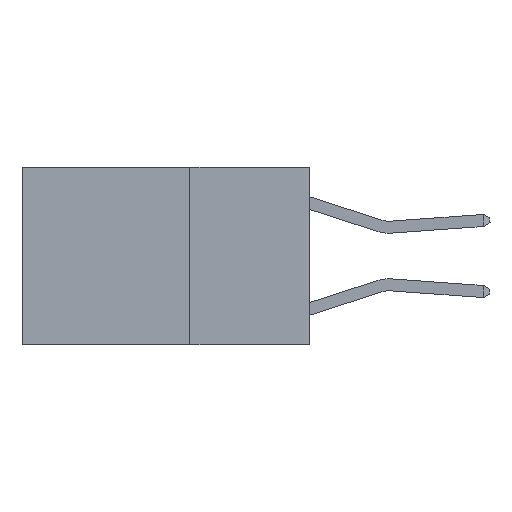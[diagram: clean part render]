
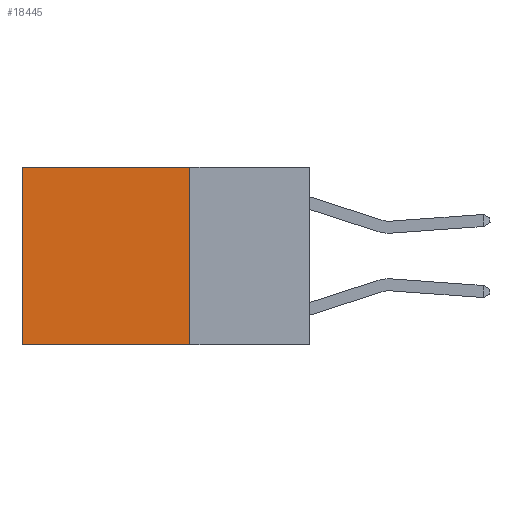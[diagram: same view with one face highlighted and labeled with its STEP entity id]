
A CAD part, left-side view. The second image highlights one B-rep face of the part: STEP entity #18445.
In plain terms, the highlighted planar face has unit normal (-1, 0, 0).
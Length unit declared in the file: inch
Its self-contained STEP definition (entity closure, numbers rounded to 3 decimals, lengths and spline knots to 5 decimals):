
#543 = LINE ( 'NONE', #3428, #13160 ) ;
#1810 = VECTOR ( 'NONE', #3182, 39.37008 ) ;
#2720 = ORIENTED_EDGE ( 'NONE', *, *, #27945, .F. ) ;
#2787 = CARTESIAN_POINT ( 'NONE',  ( 0.2625, 0.6, 0. ) ) ;
#3105 = CARTESIAN_POINT ( 'NONE',  ( 0.2625, 0.6, -0.37 ) ) ;
#3182 = DIRECTION ( 'NONE',  ( 0., 0., -1. ) ) ;
#3428 = CARTESIAN_POINT ( 'NONE',  ( 0.2625, 0.25, 0. ) ) ;
#3459 = PLANE ( 'NONE',  #4349 ) ;
#4349 = AXIS2_PLACEMENT_3D ( 'NONE', #16695, #25955, #12263 ) ;
#5688 = DIRECTION ( 'NONE',  ( 0., 1., 0. ) ) ;
#6063 = EDGE_LOOP ( 'NONE', ( #16466, #2720, #22241, #25282 ) ) ;
#7013 = LINE ( 'NONE', #18595, #1810 ) ;
#7098 = VERTEX_POINT ( 'NONE', #15454 ) ;
#8985 = CARTESIAN_POINT ( 'NONE',  ( 0.2625, 0.25, -0.37 ) ) ;
#10956 = VECTOR ( 'NONE', #25641, 39.37008 ) ;
#12170 = VERTEX_POINT ( 'NONE', #20185 ) ;
#12263 = DIRECTION ( 'NONE',  ( 0., 0., -1. ) ) ;
#12449 = EDGE_CURVE ( 'NONE', #7098, #12170, #22782, .T. ) ;
#13127 = VERTEX_POINT ( 'NONE', #3105 ) ;
#13160 = VECTOR ( 'NONE', #5688, 39.37008 ) ;
#13469 = EDGE_CURVE ( 'NONE', #22632, #13127, #7013, .T. ) ;
#14571 = FACE_OUTER_BOUND ( 'NONE', #6063, .T. ) ;
#15454 = CARTESIAN_POINT ( 'NONE',  ( 0.2625, 0.25, 0. ) ) ;
#16466 = ORIENTED_EDGE ( 'NONE', *, *, #13469, .T. ) ;
#16695 = CARTESIAN_POINT ( 'NONE',  ( 0.2625, 0.25, 0. ) ) ;
#18262 = VECTOR ( 'NONE', #27543, 39.37008 ) ;
#18445 = ADVANCED_FACE ( 'NONE', ( #14571 ), #3459, .F. ) ;
#18595 = CARTESIAN_POINT ( 'NONE',  ( 0.2625, 0.6, 0. ) ) ;
#20178 = EDGE_CURVE ( 'NONE', #7098, #22632, #543, .T. ) ;
#20185 = CARTESIAN_POINT ( 'NONE',  ( 0.2625, 0.25, -0.37 ) ) ;
#20947 = CARTESIAN_POINT ( 'NONE',  ( 0.2625, 0.25, 0. ) ) ;
#22241 = ORIENTED_EDGE ( 'NONE', *, *, #12449, .F. ) ;
#22632 = VERTEX_POINT ( 'NONE', #2787 ) ;
#22782 = LINE ( 'NONE', #20947, #10956 ) ;
#25282 = ORIENTED_EDGE ( 'NONE', *, *, #20178, .T. ) ;
#25641 = DIRECTION ( 'NONE',  ( 0., 0., -1. ) ) ;
#25955 = DIRECTION ( 'NONE',  ( 1., 0., 0. ) ) ;
#27543 = DIRECTION ( 'NONE',  ( 0., 1., 0. ) ) ;
#27945 = EDGE_CURVE ( 'NONE', #12170, #13127, #29803, .T. ) ;
#29803 = LINE ( 'NONE', #8985, #18262 ) ;
